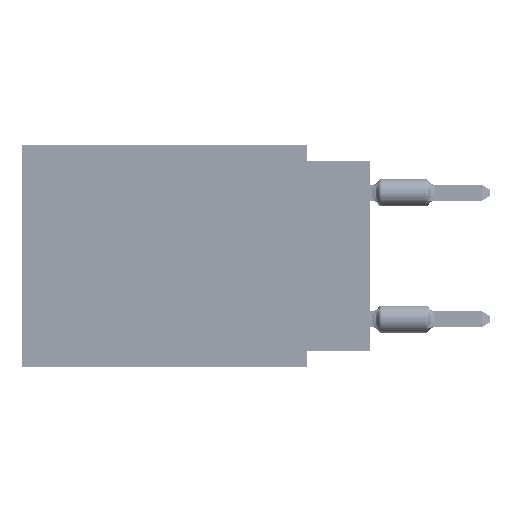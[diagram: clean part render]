
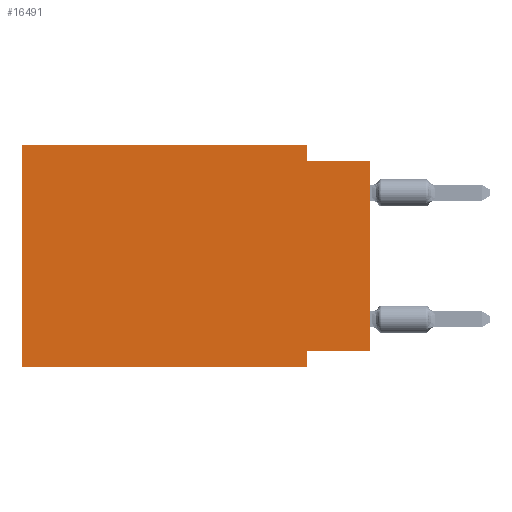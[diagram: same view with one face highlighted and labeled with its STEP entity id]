
A CAD part, left-side view. The second image highlights one B-rep face of the part: STEP entity #16491.
In plain terms, the highlighted planar face has unit normal (-1, 0, 0).
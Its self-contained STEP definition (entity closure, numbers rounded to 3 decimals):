
#2392 = DIRECTION ( 'NONE',  ( 0., 1., 0. ) ) ;
#2673 = CARTESIAN_POINT ( 'NONE',  ( 0., 0., 0. ) ) ;
#3209 = CARTESIAN_POINT ( 'NONE',  ( 0., 2.54, -8.255 ) ) ;
#3663 = ORIENTED_EDGE ( 'NONE', *, *, #41375, .F. ) ;
#6246 = CARTESIAN_POINT ( 'NONE',  ( 0., 0., -0.635 ) ) ;
#7143 = VERTEX_POINT ( 'NONE', #3209 ) ;
#9756 = EDGE_CURVE ( 'NONE', #7143, #55963, #56470, .T. ) ;
#9831 = VECTOR ( 'NONE', #2392, 1000. ) ;
#10804 = DIRECTION ( 'NONE',  ( 0., -1., 0. ) ) ;
#11309 = LINE ( 'NONE', #66148, #35345 ) ;
#11997 = VECTOR ( 'NONE', #64233, 1000. ) ;
#12184 = CARTESIAN_POINT ( 'NONE',  ( 0., 0., -8.255 ) ) ;
#14063 = VERTEX_POINT ( 'NONE', #57438 ) ;
#15233 = ORIENTED_EDGE ( 'NONE', *, *, #34712, .F. ) ;
#16205 = VERTEX_POINT ( 'NONE', #17831 ) ;
#16491 = ADVANCED_FACE ( 'NONE', ( #53910 ), #79077, .F. ) ;
#17058 = VERTEX_POINT ( 'NONE', #12184 ) ;
#17831 = CARTESIAN_POINT ( 'NONE',  ( 0., 2.54, 0. ) ) ;
#19185 = DIRECTION ( 'NONE',  ( 0., 0., -1. ) ) ;
#20572 = CARTESIAN_POINT ( 'NONE',  ( 0., 2.54, -8.89 ) ) ;
#22236 = CARTESIAN_POINT ( 'NONE',  ( 0., 13.97, 0. ) ) ;
#22414 = VECTOR ( 'NONE', #45713, 1000. ) ;
#22589 = DIRECTION ( 'NONE',  ( 1., 0., 0. ) ) ;
#24550 = VECTOR ( 'NONE', #19185, 1000. ) ;
#25232 = ORIENTED_EDGE ( 'NONE', *, *, #32087, .F. ) ;
#28722 = ORIENTED_EDGE ( 'NONE', *, *, #9756, .F. ) ;
#29845 = DIRECTION ( 'NONE',  ( 0., -1., 0. ) ) ;
#31970 = DIRECTION ( 'NONE',  ( 0., -1., 0. ) ) ;
#32087 = EDGE_CURVE ( 'NONE', #16205, #68491, #50533, .T. ) ;
#32284 = EDGE_LOOP ( 'NONE', ( #45144, #3663, #25232, #32345, #15233, #62380, #28722, #68394 ) ) ;
#32345 = ORIENTED_EDGE ( 'NONE', *, *, #65990, .F. ) ;
#34712 = EDGE_CURVE ( 'NONE', #72600, #67255, #69620, .T. ) ;
#35103 = CARTESIAN_POINT ( 'NONE',  ( 0., 2.54, -8.89 ) ) ;
#35345 = VECTOR ( 'NONE', #29845, 1000. ) ;
#38147 = CARTESIAN_POINT ( 'NONE',  ( 0., 13.97, -8.89 ) ) ;
#40192 = LINE ( 'NONE', #2673, #41928 ) ;
#41375 = EDGE_CURVE ( 'NONE', #68491, #14063, #67265, .T. ) ;
#41928 = VECTOR ( 'NONE', #76918, 1000. ) ;
#45144 = ORIENTED_EDGE ( 'NONE', *, *, #65751, .T. ) ;
#45713 = DIRECTION ( 'NONE',  ( 0., 0., -1. ) ) ;
#49709 = CARTESIAN_POINT ( 'NONE',  ( 0., 2.54, 0. ) ) ;
#50533 = LINE ( 'NONE', #49709, #24550 ) ;
#52277 = CARTESIAN_POINT ( 'NONE',  ( 0., 0., -8.255 ) ) ;
#53910 = FACE_OUTER_BOUND ( 'NONE', #32284, .T. ) ;
#55963 = VERTEX_POINT ( 'NONE', #35103 ) ;
#56470 = LINE ( 'NONE', #20572, #22414 ) ;
#57438 = CARTESIAN_POINT ( 'NONE',  ( 0., 0., -0.635 ) ) ;
#57642 = CARTESIAN_POINT ( 'NONE',  ( 0., 13.97, 0. ) ) ;
#57897 = EDGE_CURVE ( 'NONE', #17058, #7143, #70453, .T. ) ;
#61118 = AXIS2_PLACEMENT_3D ( 'NONE', #70577, #22589, #64378 ) ;
#62380 = ORIENTED_EDGE ( 'NONE', *, *, #76390, .T. ) ;
#64233 = DIRECTION ( 'NONE',  ( 0., 0., 1. ) ) ;
#64378 = DIRECTION ( 'NONE',  ( 0., 0., -1. ) ) ;
#64443 = VECTOR ( 'NONE', #31970, 1000. ) ;
#65162 = CARTESIAN_POINT ( 'NONE',  ( 0., 2.54, -0.635 ) ) ;
#65751 = EDGE_CURVE ( 'NONE', #17058, #14063, #40192, .T. ) ;
#65990 = EDGE_CURVE ( 'NONE', #67255, #16205, #11309, .T. ) ;
#66148 = CARTESIAN_POINT ( 'NONE',  ( 0., 13.97, 0. ) ) ;
#67255 = VERTEX_POINT ( 'NONE', #22236 ) ;
#67265 = LINE ( 'NONE', #6246, #68312 ) ;
#68312 = VECTOR ( 'NONE', #10804, 1000. ) ;
#68394 = ORIENTED_EDGE ( 'NONE', *, *, #57897, .F. ) ;
#68491 = VERTEX_POINT ( 'NONE', #65162 ) ;
#69620 = LINE ( 'NONE', #57642, #11997 ) ;
#70453 = LINE ( 'NONE', #52277, #9831 ) ;
#70577 = CARTESIAN_POINT ( 'NONE',  ( 0., 13.97, 0. ) ) ;
#70710 = LINE ( 'NONE', #38147, #64443 ) ;
#72600 = VERTEX_POINT ( 'NONE', #81505 ) ;
#76390 = EDGE_CURVE ( 'NONE', #72600, #55963, #70710, .T. ) ;
#76918 = DIRECTION ( 'NONE',  ( 0., 0., 1. ) ) ;
#79077 = PLANE ( 'NONE',  #61118 ) ;
#81505 = CARTESIAN_POINT ( 'NONE',  ( 0., 13.97, -8.89 ) ) ;
